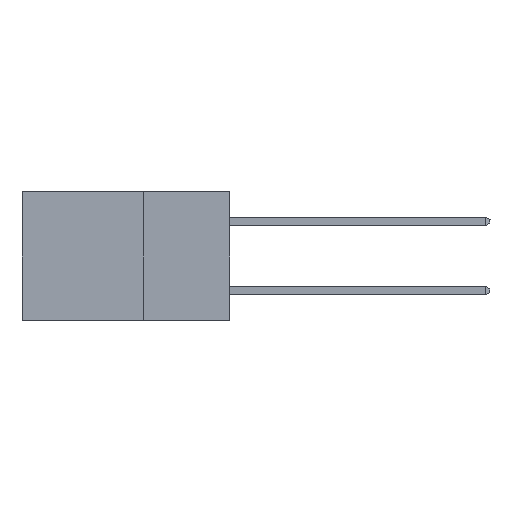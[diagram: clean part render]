
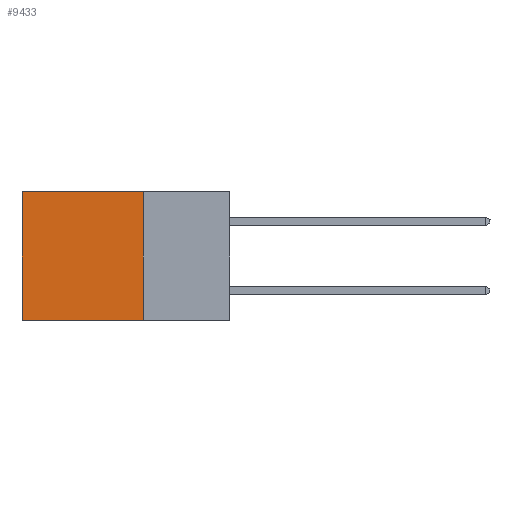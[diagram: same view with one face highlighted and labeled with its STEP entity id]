
A CAD part, left-side view. The second image highlights one B-rep face of the part: STEP entity #9433.
In plain terms, the highlighted planar face has unit normal (-1, 0, 0).
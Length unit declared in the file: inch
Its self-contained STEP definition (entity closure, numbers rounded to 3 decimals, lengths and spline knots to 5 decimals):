
#528 = CARTESIAN_POINT ( 'NONE',  ( 0.2615, 0.6, -0.37 ) ) ;
#1087 = ORIENTED_EDGE ( 'NONE', *, *, #3850, .F. ) ;
#1251 = CARTESIAN_POINT ( 'NONE',  ( 0.2615, 0.25, -0.37 ) ) ;
#1584 = DIRECTION ( 'NONE',  ( 0., 1., 0. ) ) ;
#1591 = VERTEX_POINT ( 'NONE', #4292 ) ;
#1630 = VERTEX_POINT ( 'NONE', #8362 ) ;
#1639 = LINE ( 'NONE', #9145, #2209 ) ;
#2151 = EDGE_CURVE ( 'NONE', #1591, #8635, #6887, .T. ) ;
#2209 = VECTOR ( 'NONE', #8185, 39.37008 ) ;
#2210 = DIRECTION ( 'NONE',  ( 0., 0., -1. ) ) ;
#2264 = LINE ( 'NONE', #528, #6752 ) ;
#2523 = EDGE_LOOP ( 'NONE', ( #9699, #1087, #8910, #8809 ) ) ;
#3171 = PLANE ( 'NONE',  #4216 ) ;
#3850 = EDGE_CURVE ( 'NONE', #8635, #1630, #1639, .T. ) ;
#3859 = DIRECTION ( 'NONE',  ( 0., 0., -1. ) ) ;
#4216 = AXIS2_PLACEMENT_3D ( 'NONE', #7937, #9763, #3859 ) ;
#4292 = CARTESIAN_POINT ( 'NONE',  ( 0.2615, 0.25, 0. ) ) ;
#4815 = CARTESIAN_POINT ( 'NONE',  ( 0.2615, 0.25, 0. ) ) ;
#5484 = VERTEX_POINT ( 'NONE', #8184 ) ;
#5498 = EDGE_CURVE ( 'NONE', #1591, #5484, #7970, .T. ) ;
#5890 = VECTOR ( 'NONE', #1584, 39.37008 ) ;
#6303 = EDGE_CURVE ( 'NONE', #5484, #1630, #2264, .T. ) ;
#6752 = VECTOR ( 'NONE', #2210, 39.37008 ) ;
#6887 = LINE ( 'NONE', #1251, #8440 ) ;
#7002 = DIRECTION ( 'NONE',  ( 0., 0., -1. ) ) ;
#7233 = FACE_OUTER_BOUND ( 'NONE', #2523, .T. ) ;
#7937 = CARTESIAN_POINT ( 'NONE',  ( 0.2615, 0.25, -0.37 ) ) ;
#7970 = LINE ( 'NONE', #4815, #5890 ) ;
#8184 = CARTESIAN_POINT ( 'NONE',  ( 0.2615, 0.6, 0. ) ) ;
#8185 = DIRECTION ( 'NONE',  ( 0., 1., 0. ) ) ;
#8362 = CARTESIAN_POINT ( 'NONE',  ( 0.2615, 0.6, -0.37 ) ) ;
#8440 = VECTOR ( 'NONE', #7002, 39.37008 ) ;
#8635 = VERTEX_POINT ( 'NONE', #9147 ) ;
#8809 = ORIENTED_EDGE ( 'NONE', *, *, #5498, .T. ) ;
#8910 = ORIENTED_EDGE ( 'NONE', *, *, #2151, .F. ) ;
#9145 = CARTESIAN_POINT ( 'NONE',  ( 0.2615, 0.25, -0.37 ) ) ;
#9147 = CARTESIAN_POINT ( 'NONE',  ( 0.2615, 0.25, -0.37 ) ) ;
#9433 = ADVANCED_FACE ( 'NONE', ( #7233 ), #3171, .F. ) ;
#9699 = ORIENTED_EDGE ( 'NONE', *, *, #6303, .T. ) ;
#9763 = DIRECTION ( 'NONE',  ( 1., 0., 0. ) ) ;
